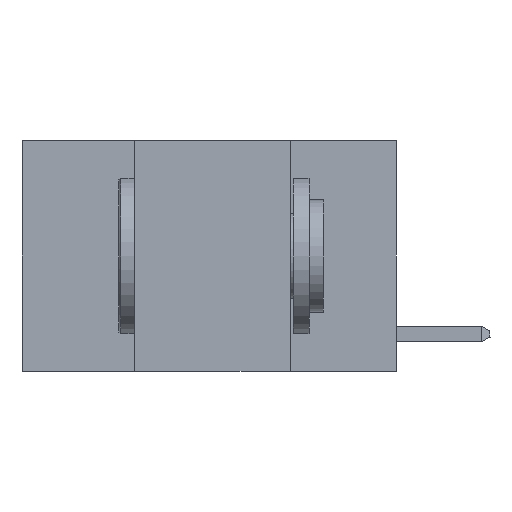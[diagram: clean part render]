
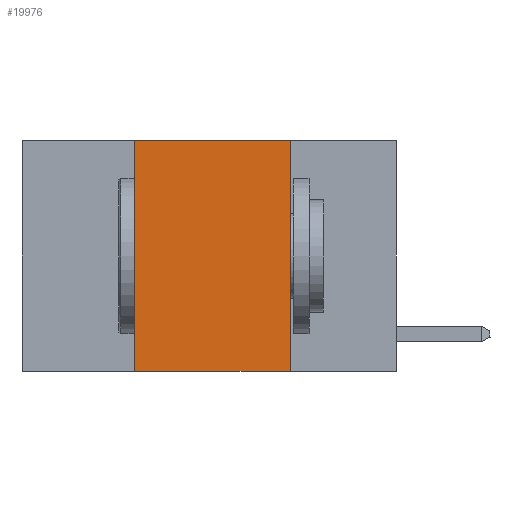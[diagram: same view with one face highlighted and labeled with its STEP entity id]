
A CAD part, left-side view. The second image highlights one B-rep face of the part: STEP entity #19976.
In plain terms, the highlighted planar face has unit normal (-1, 0, 0).
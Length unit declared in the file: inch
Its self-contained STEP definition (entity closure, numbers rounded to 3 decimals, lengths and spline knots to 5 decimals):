
#811 = CARTESIAN_POINT ( 'NONE',  ( 0., 0.6, -0.37 ) ) ;
#1515 = LINE ( 'NONE', #15786, #21952 ) ;
#3855 = VECTOR ( 'NONE', #8216, 39.37008 ) ;
#4267 = CARTESIAN_POINT ( 'NONE',  ( 0., 0.42, -0.37 ) ) ;
#4296 = DIRECTION ( 'NONE',  ( 0., 0., -1. ) ) ;
#5598 = EDGE_LOOP ( 'NONE', ( #11204, #22948, #25373, #24938 ) ) ;
#5846 = AXIS2_PLACEMENT_3D ( 'NONE', #16634, #26638, #24480 ) ;
#7760 = CARTESIAN_POINT ( 'NONE',  ( 0., 0.17, -0.37 ) ) ;
#8216 = DIRECTION ( 'NONE',  ( 0., -1., 0. ) ) ;
#11204 = ORIENTED_EDGE ( 'NONE', *, *, #13120, .F. ) ;
#12721 = CARTESIAN_POINT ( 'NONE',  ( 0., 0.17, 0. ) ) ;
#13120 = EDGE_CURVE ( 'NONE', #20491, #15651, #15026, .T. ) ;
#14843 = VERTEX_POINT ( 'NONE', #4267 ) ;
#15026 = LINE ( 'NONE', #12721, #22082 ) ;
#15651 = VERTEX_POINT ( 'NONE', #7760 ) ;
#15786 = CARTESIAN_POINT ( 'NONE',  ( 0., 0.42, 0. ) ) ;
#16363 = LINE ( 'NONE', #22736, #3855 ) ;
#16634 = CARTESIAN_POINT ( 'NONE',  ( 0., 0.6, 0. ) ) ;
#16854 = CARTESIAN_POINT ( 'NONE',  ( 0., 0.42, 0. ) ) ;
#16952 = VECTOR ( 'NONE', #23356, 39.37008 ) ;
#17500 = VERTEX_POINT ( 'NONE', #16854 ) ;
#18259 = PLANE ( 'NONE',  #5846 ) ;
#19092 = CARTESIAN_POINT ( 'NONE',  ( 0., 0.17, 0. ) ) ;
#19558 = LINE ( 'NONE', #811, #16952 ) ;
#19976 = ADVANCED_FACE ( 'NONE', ( #20706 ), #18259, .F. ) ;
#20491 = VERTEX_POINT ( 'NONE', #19092 ) ;
#20706 = FACE_OUTER_BOUND ( 'NONE', #5598, .T. ) ;
#21952 = VECTOR ( 'NONE', #22151, 39.37008 ) ;
#22082 = VECTOR ( 'NONE', #4296, 39.37008 ) ;
#22151 = DIRECTION ( 'NONE',  ( 0., 0., 1. ) ) ;
#22497 = EDGE_CURVE ( 'NONE', #14843, #17500, #1515, .T. ) ;
#22736 = CARTESIAN_POINT ( 'NONE',  ( 0., 0.6, 0. ) ) ;
#22948 = ORIENTED_EDGE ( 'NONE', *, *, #24463, .F. ) ;
#23356 = DIRECTION ( 'NONE',  ( 0., -1., 0. ) ) ;
#24078 = EDGE_CURVE ( 'NONE', #14843, #15651, #19558, .T. ) ;
#24463 = EDGE_CURVE ( 'NONE', #17500, #20491, #16363, .T. ) ;
#24480 = DIRECTION ( 'NONE',  ( 0., 0., -1. ) ) ;
#24938 = ORIENTED_EDGE ( 'NONE', *, *, #24078, .T. ) ;
#25373 = ORIENTED_EDGE ( 'NONE', *, *, #22497, .F. ) ;
#26638 = DIRECTION ( 'NONE',  ( 1., 0., 0. ) ) ;
